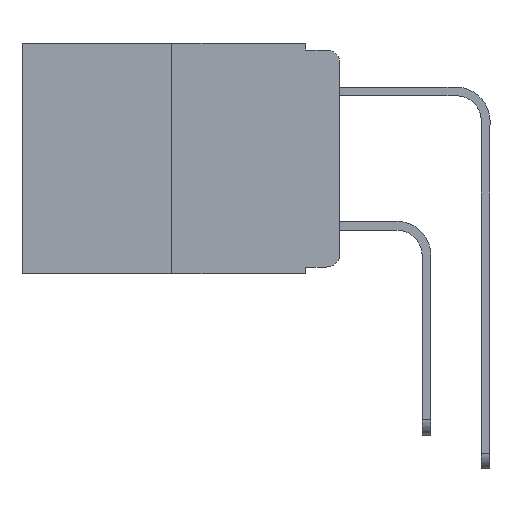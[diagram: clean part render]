
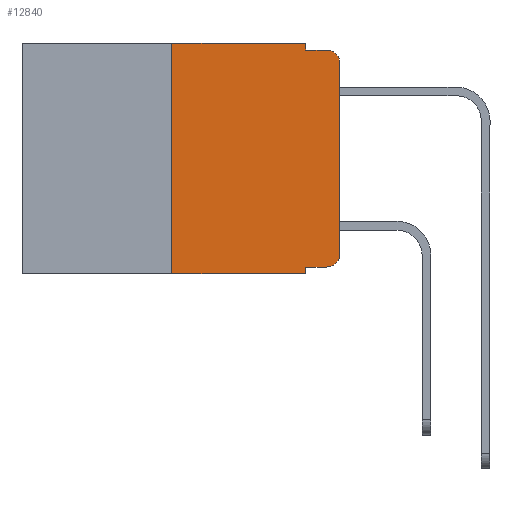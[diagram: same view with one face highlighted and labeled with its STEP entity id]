
A CAD part, left-side view. The second image highlights one B-rep face of the part: STEP entity #12840.
In plain terms, the highlighted planar face has unit normal (-1, 0, 0).
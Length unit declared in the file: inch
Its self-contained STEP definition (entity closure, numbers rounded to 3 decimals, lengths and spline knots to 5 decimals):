
#93 = AXIS2_PLACEMENT_3D ( 'NONE', #3745, #7021, #497 ) ;
#146 = VERTEX_POINT ( 'NONE', #7145 ) ;
#497 = DIRECTION ( 'NONE',  ( 0., 0., -1. ) ) ;
#637 = VECTOR ( 'NONE', #8761, 39.37008 ) ;
#717 = LINE ( 'NONE', #11496, #6193 ) ;
#1189 = CARTESIAN_POINT ( 'NONE',  ( 0., 0.051, 0. ) ) ;
#1240 = ORIENTED_EDGE ( 'NONE', *, *, #5780, .F. ) ;
#1280 = CARTESIAN_POINT ( 'NONE',  ( 0., 0.02, -0.03 ) ) ;
#1315 = ORIENTED_EDGE ( 'NONE', *, *, #2228, .T. ) ;
#1367 = EDGE_CURVE ( 'NONE', #12852, #2284, #8698, .T. ) ;
#1497 = EDGE_LOOP ( 'NONE', ( #11730, #9631, #2821, #2345, #10799, #1240, #2939, #8788, #1315, #4526 ) ) ;
#2033 = CARTESIAN_POINT ( 'NONE',  ( 0., 0.25, -0.343 ) ) ;
#2088 = VERTEX_POINT ( 'NONE', #2033 ) ;
#2156 = DIRECTION ( 'NONE',  ( 0., 0., 1. ) ) ;
#2228 = EDGE_CURVE ( 'NONE', #146, #13419, #8149, .T. ) ;
#2284 = VERTEX_POINT ( 'NONE', #10645 ) ;
#2345 = ORIENTED_EDGE ( 'NONE', *, *, #9247, .F. ) ;
#2385 = DIRECTION ( 'NONE',  ( 0., 0., -1. ) ) ;
#2396 = VECTOR ( 'NONE', #4205, 39.37008 ) ;
#2421 = LINE ( 'NONE', #9671, #4938 ) ;
#2501 = CIRCLE ( 'NONE', #5515, 0.02 ) ;
#2613 = LINE ( 'NONE', #12108, #8017 ) ;
#2821 = ORIENTED_EDGE ( 'NONE', *, *, #1367, .F. ) ;
#2939 = ORIENTED_EDGE ( 'NONE', *, *, #11494, .T. ) ;
#3011 = DIRECTION ( 'NONE',  ( 0., 0., -1. ) ) ;
#3707 = CARTESIAN_POINT ( 'NONE',  ( 0., 0.02, -0.313 ) ) ;
#3745 = CARTESIAN_POINT ( 'NONE',  ( 0., 0.473, 0. ) ) ;
#3805 = VERTEX_POINT ( 'NONE', #3893 ) ;
#3893 = CARTESIAN_POINT ( 'NONE',  ( 0., 0.051, -0.343 ) ) ;
#3927 = VERTEX_POINT ( 'NONE', #10653 ) ;
#4205 = DIRECTION ( 'NONE',  ( 0., -1., 0. ) ) ;
#4423 = CIRCLE ( 'NONE', #7910, 0.02 ) ;
#4526 = ORIENTED_EDGE ( 'NONE', *, *, #10238, .T. ) ;
#4775 = DIRECTION ( 'NONE',  ( 0., 0., -1. ) ) ;
#4820 = CARTESIAN_POINT ( 'NONE',  ( 0., 0.051, 0. ) ) ;
#4851 = VERTEX_POINT ( 'NONE', #13137 ) ;
#4938 = VECTOR ( 'NONE', #2156, 39.37008 ) ;
#4981 = CARTESIAN_POINT ( 'NONE',  ( 0., 0.473, -0.343 ) ) ;
#5354 = EDGE_CURVE ( 'NONE', #13300, #2284, #2501, .T. ) ;
#5461 = CARTESIAN_POINT ( 'NONE',  ( 0., 0.051, -0.01 ) ) ;
#5515 = AXIS2_PLACEMENT_3D ( 'NONE', #1280, #8846, #2385 ) ;
#5561 = DIRECTION ( 'NONE',  ( 0., -1., 0. ) ) ;
#5726 = VECTOR ( 'NONE', #7342, 39.37008 ) ;
#5780 = EDGE_CURVE ( 'NONE', #2088, #4851, #6408, .T. ) ;
#6069 = DIRECTION ( 'NONE',  ( 0., -1., 0. ) ) ;
#6172 = CARTESIAN_POINT ( 'NONE',  ( 0., 0.02, -0.333 ) ) ;
#6193 = VECTOR ( 'NONE', #3011, 39.37008 ) ;
#6408 = LINE ( 'NONE', #12494, #5726 ) ;
#6592 = FACE_OUTER_BOUND ( 'NONE', #1497, .T. ) ;
#6963 = DIRECTION ( 'NONE',  ( 0., -1., 0. ) ) ;
#7021 = DIRECTION ( 'NONE',  ( 1., 0., 0. ) ) ;
#7145 = CARTESIAN_POINT ( 'NONE',  ( 0., 0.051, -0.333 ) ) ;
#7342 = DIRECTION ( 'NONE',  ( 0., 0., 1. ) ) ;
#7431 = CARTESIAN_POINT ( 'NONE',  ( 0., 0.051, -0.333 ) ) ;
#7910 = AXIS2_PLACEMENT_3D ( 'NONE', #3707, #11110, #4775 ) ;
#8017 = VECTOR ( 'NONE', #6963, 39.37008 ) ;
#8149 = LINE ( 'NONE', #7431, #2396 ) ;
#8641 = EDGE_CURVE ( 'NONE', #4851, #10274, #2613, .T. ) ;
#8698 = LINE ( 'NONE', #5461, #11406 ) ;
#8761 = DIRECTION ( 'NONE',  ( 0., 0., -1. ) ) ;
#8788 = ORIENTED_EDGE ( 'NONE', *, *, #11805, .F. ) ;
#8846 = DIRECTION ( 'NONE',  ( -1., 0., 0. ) ) ;
#9162 = CARTESIAN_POINT ( 'NONE',  ( 0., 0.051, -0.01 ) ) ;
#9247 = EDGE_CURVE ( 'NONE', #10274, #12852, #717, .T. ) ;
#9631 = ORIENTED_EDGE ( 'NONE', *, *, #5354, .T. ) ;
#9671 = CARTESIAN_POINT ( 'NONE',  ( 0., 0., 0. ) ) ;
#9995 = EDGE_CURVE ( 'NONE', #3927, #13300, #2421, .T. ) ;
#10238 = EDGE_CURVE ( 'NONE', #13419, #3927, #4423, .T. ) ;
#10274 = VERTEX_POINT ( 'NONE', #4820 ) ;
#10645 = CARTESIAN_POINT ( 'NONE',  ( 0., 0.02, -0.01 ) ) ;
#10653 = CARTESIAN_POINT ( 'NONE',  ( 0., 0., -0.313 ) ) ;
#10799 = ORIENTED_EDGE ( 'NONE', *, *, #8641, .F. ) ;
#11110 = DIRECTION ( 'NONE',  ( -1., 0., 0. ) ) ;
#11406 = VECTOR ( 'NONE', #5561, 39.37008 ) ;
#11494 = EDGE_CURVE ( 'NONE', #2088, #3805, #13690, .T. ) ;
#11496 = CARTESIAN_POINT ( 'NONE',  ( 0., 0.051, 0. ) ) ;
#11730 = ORIENTED_EDGE ( 'NONE', *, *, #9995, .T. ) ;
#11805 = EDGE_CURVE ( 'NONE', #146, #3805, #11966, .T. ) ;
#11966 = LINE ( 'NONE', #1189, #637 ) ;
#12108 = CARTESIAN_POINT ( 'NONE',  ( 0., 0.473, 0. ) ) ;
#12173 = PLANE ( 'NONE',  #93 ) ;
#12494 = CARTESIAN_POINT ( 'NONE',  ( 0., 0.25, 0. ) ) ;
#12840 = ADVANCED_FACE ( 'NONE', ( #6592 ), #12173, .F. ) ;
#12852 = VERTEX_POINT ( 'NONE', #9162 ) ;
#12941 = CARTESIAN_POINT ( 'NONE',  ( 0., 0., -0.03 ) ) ;
#13101 = VECTOR ( 'NONE', #6069, 39.37008 ) ;
#13137 = CARTESIAN_POINT ( 'NONE',  ( 0., 0.25, 0. ) ) ;
#13300 = VERTEX_POINT ( 'NONE', #12941 ) ;
#13419 = VERTEX_POINT ( 'NONE', #6172 ) ;
#13690 = LINE ( 'NONE', #4981, #13101 ) ;
